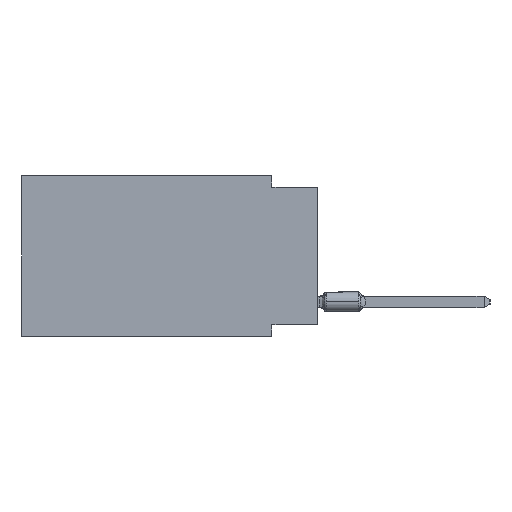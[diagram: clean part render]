
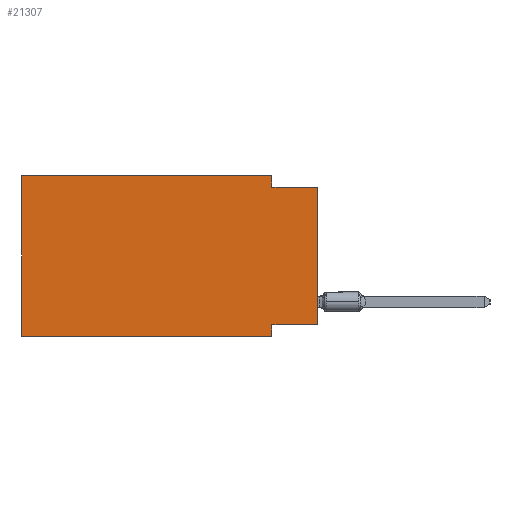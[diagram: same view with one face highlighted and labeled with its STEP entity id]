
A CAD part, left-side view. The second image highlights one B-rep face of the part: STEP entity #21307.
In plain terms, the highlighted planar face has unit normal (-1, 0, 0).
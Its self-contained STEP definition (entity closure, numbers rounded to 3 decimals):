
#78 = VECTOR ( 'NONE', #27791, 1000. ) ;
#804 = VECTOR ( 'NONE', #21229, 1000. ) ;
#1914 = ORIENTED_EDGE ( 'NONE', *, *, #9678, .F. ) ;
#1918 = VECTOR ( 'NONE', #35858, 1000. ) ;
#3133 = CARTESIAN_POINT ( 'NONE',  ( 0., 0., -8.255 ) ) ;
#3524 = CARTESIAN_POINT ( 'NONE',  ( 0., 2.54, 0. ) ) ;
#4080 = PLANE ( 'NONE',  #28032 ) ;
#4696 = LINE ( 'NONE', #36400, #1918 ) ;
#4943 = CARTESIAN_POINT ( 'NONE',  ( 0., 16.383, 0. ) ) ;
#5995 = VERTEX_POINT ( 'NONE', #15919 ) ;
#6033 = ORIENTED_EDGE ( 'NONE', *, *, #9749, .F. ) ;
#7040 = DIRECTION ( 'NONE',  ( 0., 0., -1. ) ) ;
#7085 = VERTEX_POINT ( 'NONE', #23538 ) ;
#8197 = VERTEX_POINT ( 'NONE', #9821 ) ;
#8785 = CARTESIAN_POINT ( 'NONE',  ( 0., 16.383, -8.89 ) ) ;
#8788 = ORIENTED_EDGE ( 'NONE', *, *, #36471, .F. ) ;
#8840 = LINE ( 'NONE', #22573, #22081 ) ;
#8956 = ORIENTED_EDGE ( 'NONE', *, *, #12890, .T. ) ;
#9678 = EDGE_CURVE ( 'NONE', #34553, #29728, #18680, .T. ) ;
#9749 = EDGE_CURVE ( 'NONE', #5995, #7085, #13636, .T. ) ;
#9821 = CARTESIAN_POINT ( 'NONE',  ( 0., 2.54, -8.89 ) ) ;
#12075 = VECTOR ( 'NONE', #34281, 1000. ) ;
#12479 = CARTESIAN_POINT ( 'NONE',  ( 0., 0., -8.255 ) ) ;
#12890 = EDGE_CURVE ( 'NONE', #34332, #8197, #28272, .T. ) ;
#13461 = CARTESIAN_POINT ( 'NONE',  ( 0., 16.383, -8.89 ) ) ;
#13636 = LINE ( 'NONE', #16437, #13827 ) ;
#13827 = VECTOR ( 'NONE', #30868, 1000. ) ;
#15066 = VERTEX_POINT ( 'NONE', #23372 ) ;
#15593 = VECTOR ( 'NONE', #15709, 1000. ) ;
#15709 = DIRECTION ( 'NONE',  ( 0., -1., 0. ) ) ;
#15919 = CARTESIAN_POINT ( 'NONE',  ( 0., 2.54, -0.635 ) ) ;
#16437 = CARTESIAN_POINT ( 'NONE',  ( 0., 0., -0.635 ) ) ;
#18680 = LINE ( 'NONE', #4943, #15593 ) ;
#19124 = EDGE_CURVE ( 'NONE', #29728, #5995, #30741, .T. ) ;
#20426 = CARTESIAN_POINT ( 'NONE',  ( 0., 16.383, 0. ) ) ;
#20766 = DIRECTION ( 'NONE',  ( 1., 0., 0. ) ) ;
#21229 = DIRECTION ( 'NONE',  ( 0., 0., 1. ) ) ;
#21307 = ADVANCED_FACE ( 'NONE', ( #29112 ), #4080, .F. ) ;
#21659 = EDGE_CURVE ( 'NONE', #36297, #15066, #36335, .T. ) ;
#22081 = VECTOR ( 'NONE', #28692, 1000. ) ;
#22573 = CARTESIAN_POINT ( 'NONE',  ( 0., 16.383, 0. ) ) ;
#23372 = CARTESIAN_POINT ( 'NONE',  ( 0., 2.54, -8.255 ) ) ;
#23538 = CARTESIAN_POINT ( 'NONE',  ( 0., 0., -0.635 ) ) ;
#24013 = CARTESIAN_POINT ( 'NONE',  ( 0., 0., 0. ) ) ;
#24121 = ORIENTED_EDGE ( 'NONE', *, *, #28784, .F. ) ;
#24762 = ORIENTED_EDGE ( 'NONE', *, *, #21659, .F. ) ;
#26025 = CARTESIAN_POINT ( 'NONE',  ( 0., 16.383, 0. ) ) ;
#27103 = VECTOR ( 'NONE', #36064, 1000. ) ;
#27791 = DIRECTION ( 'NONE',  ( 0., 0., -1. ) ) ;
#28032 = AXIS2_PLACEMENT_3D ( 'NONE', #20426, #20766, #7040 ) ;
#28272 = LINE ( 'NONE', #13461, #27103 ) ;
#28692 = DIRECTION ( 'NONE',  ( 0., 0., 1. ) ) ;
#28784 = EDGE_CURVE ( 'NONE', #34332, #34553, #8840, .T. ) ;
#29112 = FACE_OUTER_BOUND ( 'NONE', #34834, .T. ) ;
#29198 = LINE ( 'NONE', #24013, #804 ) ;
#29728 = VERTEX_POINT ( 'NONE', #3524 ) ;
#29799 = ORIENTED_EDGE ( 'NONE', *, *, #31761, .T. ) ;
#30032 = CARTESIAN_POINT ( 'NONE',  ( 0., 2.54, 0. ) ) ;
#30741 = LINE ( 'NONE', #30032, #78 ) ;
#30868 = DIRECTION ( 'NONE',  ( 0., -1., 0. ) ) ;
#31761 = EDGE_CURVE ( 'NONE', #36297, #7085, #29198, .T. ) ;
#34281 = DIRECTION ( 'NONE',  ( 0., 1., 0. ) ) ;
#34332 = VERTEX_POINT ( 'NONE', #8785 ) ;
#34482 = ORIENTED_EDGE ( 'NONE', *, *, #19124, .F. ) ;
#34553 = VERTEX_POINT ( 'NONE', #26025 ) ;
#34834 = EDGE_LOOP ( 'NONE', ( #29799, #6033, #34482, #1914, #24121, #8956, #8788, #24762 ) ) ;
#35858 = DIRECTION ( 'NONE',  ( 0., 0., -1. ) ) ;
#36064 = DIRECTION ( 'NONE',  ( 0., -1., 0. ) ) ;
#36297 = VERTEX_POINT ( 'NONE', #12479 ) ;
#36335 = LINE ( 'NONE', #3133, #12075 ) ;
#36400 = CARTESIAN_POINT ( 'NONE',  ( 0., 2.54, -8.89 ) ) ;
#36471 = EDGE_CURVE ( 'NONE', #15066, #8197, #4696, .T. ) ;
